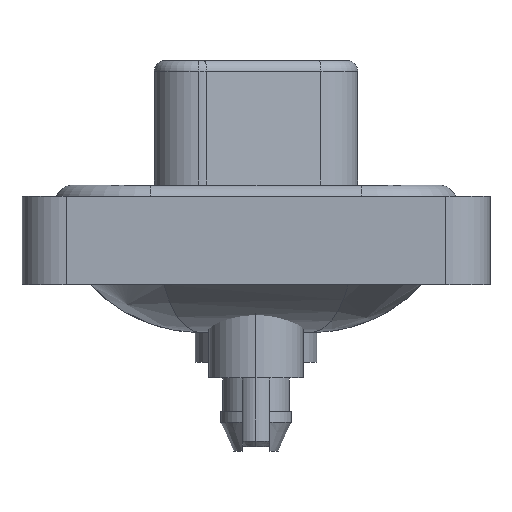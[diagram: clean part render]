
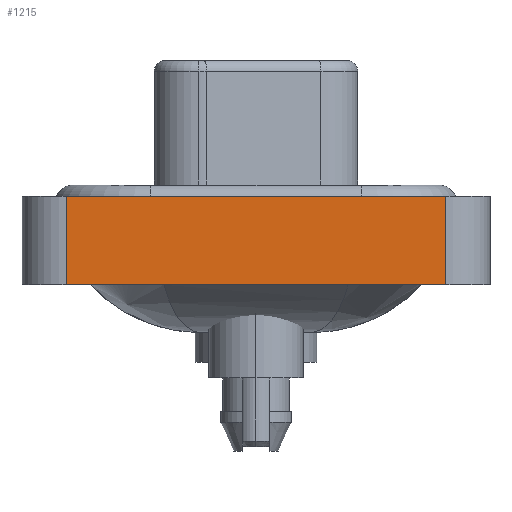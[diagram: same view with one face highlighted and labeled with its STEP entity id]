
A CAD part, left-side view. The second image highlights one B-rep face of the part: STEP entity #1215.
In plain terms, the highlighted planar face has unit normal (-1, 0, 0).
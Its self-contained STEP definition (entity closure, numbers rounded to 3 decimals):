
#2 = CARTESIAN_POINT ( 'NONE',  ( -7.3, -8.55, -3.6 ) ) ;
#797 = LINE ( 'NONE', #17017, #12638 ) ;
#1215 = ADVANCED_FACE ( 'NONE', ( #6409 ), #14391, .T. ) ;
#1627 = VERTEX_POINT ( 'NONE', #15673 ) ;
#1667 = LINE ( 'NONE', #2, #7109 ) ;
#1836 = LINE ( 'NONE', #5798, #7653 ) ;
#2451 = DIRECTION ( 'NONE',  ( -1., 0., 0. ) ) ;
#2564 = CARTESIAN_POINT ( 'NONE',  ( -7.3, 8.55, -3.6 ) ) ;
#2714 = DIRECTION ( 'NONE',  ( 0., 0., 1. ) ) ;
#2756 = VERTEX_POINT ( 'NONE', #7536 ) ;
#3112 = EDGE_CURVE ( 'NONE', #2756, #1627, #1836, .T. ) ;
#3688 = CARTESIAN_POINT ( 'NONE',  ( -7.3, -8.55, -3.6 ) ) ;
#3740 = ORIENTED_EDGE ( 'NONE', *, *, #12751, .T. ) ;
#3806 = ORIENTED_EDGE ( 'NONE', *, *, #14146, .T. ) ;
#5439 = DIRECTION ( 'NONE',  ( 0., -1., 0. ) ) ;
#5469 = EDGE_LOOP ( 'NONE', ( #3806, #12892, #11795, #3740 ) ) ;
#5798 = CARTESIAN_POINT ( 'NONE',  ( -7.3, -8.55, 0.4 ) ) ;
#6193 = AXIS2_PLACEMENT_3D ( 'NONE', #10616, #2451, #7891 ) ;
#6409 = FACE_OUTER_BOUND ( 'NONE', #5469, .T. ) ;
#7109 = VECTOR ( 'NONE', #2714, 1000. ) ;
#7514 = LINE ( 'NONE', #2564, #11546 ) ;
#7536 = CARTESIAN_POINT ( 'NONE',  ( -7.3, 8.55, 0.4 ) ) ;
#7653 = VECTOR ( 'NONE', #5439, 1000. ) ;
#7891 = DIRECTION ( 'NONE',  ( 0., 0., 1. ) ) ;
#7917 = DIRECTION ( 'NONE',  ( 0., 0., 1. ) ) ;
#10616 = CARTESIAN_POINT ( 'NONE',  ( -7.3, -8.55, -3.6 ) ) ;
#10700 = VERTEX_POINT ( 'NONE', #3688 ) ;
#11282 = EDGE_CURVE ( 'NONE', #15363, #2756, #7514, .T. ) ;
#11546 = VECTOR ( 'NONE', #7917, 1000. ) ;
#11795 = ORIENTED_EDGE ( 'NONE', *, *, #11282, .F. ) ;
#12638 = VECTOR ( 'NONE', #15775, 1000. ) ;
#12751 = EDGE_CURVE ( 'NONE', #15363, #10700, #797, .T. ) ;
#12892 = ORIENTED_EDGE ( 'NONE', *, *, #3112, .F. ) ;
#14146 = EDGE_CURVE ( 'NONE', #10700, #1627, #1667, .T. ) ;
#14391 = PLANE ( 'NONE',  #6193 ) ;
#15363 = VERTEX_POINT ( 'NONE', #16217 ) ;
#15673 = CARTESIAN_POINT ( 'NONE',  ( -7.3, -8.55, 0.4 ) ) ;
#15775 = DIRECTION ( 'NONE',  ( 0., -1., 0. ) ) ;
#16217 = CARTESIAN_POINT ( 'NONE',  ( -7.3, 8.55, -3.6 ) ) ;
#17017 = CARTESIAN_POINT ( 'NONE',  ( -7.3, -8.55, -3.6 ) ) ;
